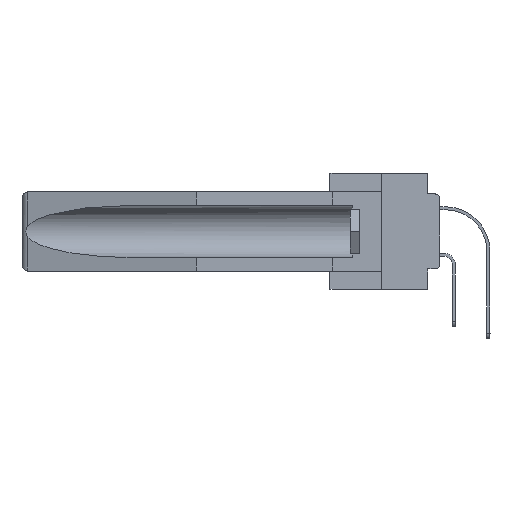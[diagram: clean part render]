
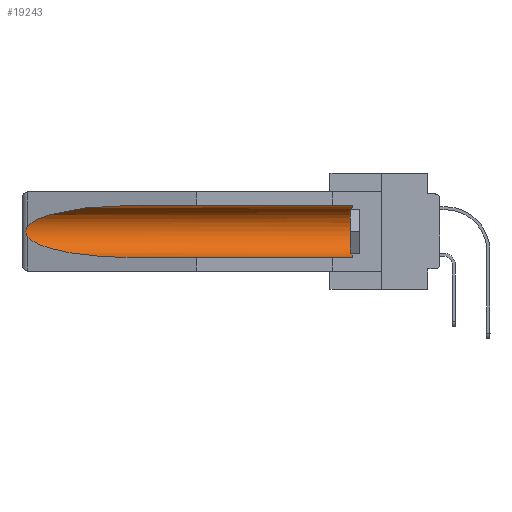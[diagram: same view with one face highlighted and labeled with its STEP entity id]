
A CAD part, left-side view. The second image highlights one B-rep face of the part: STEP entity #19243.
In plain terms, the highlighted cylindrical face has radius 2.857 mm (diameter 5.715 mm), a partial arc.
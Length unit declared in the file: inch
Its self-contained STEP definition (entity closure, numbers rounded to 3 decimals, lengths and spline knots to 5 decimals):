
#1200 = CARTESIAN_POINT ( 'NONE',  ( 0.155, 1.07973, -0.284 ) ) ;
#1222 = CARTESIAN_POINT ( 'NONE',  ( 0.2675, 1.53308, -0.16763 ) ) ;
#1404 = CARTESIAN_POINT ( 'NONE',  ( 0.26597, 1.5296, -0.19026 ) ) ;
#3200 = CARTESIAN_POINT ( 'NONE',  ( 0.26537, 1.52718, -0.19328 ) ) ;
#3252 = AXIS2_PLACEMENT_3D ( 'NONE', #8581, #19879, #29312 ) ;
#3478 =( BOUNDED_CURVE ( )  B_SPLINE_CURVE ( 3, ( #15281, #17588, #27032, #1200 ),
 .UNSPECIFIED., .F., .F. ) 
 B_SPLINE_CURVE_WITH_KNOTS ( ( 4, 4 ),
 ( 0.1948, 1.5708 ),
 .UNSPECIFIED. ) 
 CURVE ( )  GEOMETRIC_REPRESENTATION_ITEM ( )  RATIONAL_B_SPLINE_CURVE ( ( 1., 0.848, 0.848, 1. ) ) 
 REPRESENTATION_ITEM ( '' )  );
#4087 = CARTESIAN_POINT ( 'NONE',  ( 0.25451, 1.48313, -0.09465 ) ) ;
#4422 = AXIS2_PLACEMENT_3D ( 'NONE', #6371, #16258, #25703 ) ;
#4502 = EDGE_LOOP ( 'NONE', ( #12673, #25443, #23238, #27406, #7830, #9350 ) ) ;
#5231 = VECTOR ( 'NONE', #22722, 39.37008 ) ;
#5834 = LINE ( 'NONE', #6122, #15547 ) ;
#6122 = CARTESIAN_POINT ( 'NONE',  ( 0.155, -0.30754, -0.059 ) ) ;
#6148 = CARTESIAN_POINT ( 'NONE',  ( 0.155, -0.30754, -0.284 ) ) ;
#6371 = CARTESIAN_POINT ( 'NONE',  ( 0.155, -0.30754, -0.1715 ) ) ;
#6819 = CYLINDRICAL_SURFACE ( 'NONE', #4422, 0.1125 ) ;
#7031 = VERTEX_POINT ( 'NONE', #27412 ) ;
#7830 = ORIENTED_EDGE ( 'NONE', *, *, #12234, .T. ) ;
#7879 = CARTESIAN_POINT ( 'NONE',  ( 0.26537, 1.52718, -0.19328 ) ) ;
#8014 = VERTEX_POINT ( 'NONE', #3200 ) ;
#8350 = CARTESIAN_POINT ( 'NONE',  ( 0.2675, 1.53308, -0.17534 ) ) ;
#8578 = CARTESIAN_POINT ( 'NONE',  ( 0.155, 1.07973, -0.059 ) ) ;
#8581 = CARTESIAN_POINT ( 'NONE',  ( 0.155, 0.126, -0.1715 ) ) ;
#9350 = ORIENTED_EDGE ( 'NONE', *, *, #28765, .T. ) ;
#9729 = VERTEX_POINT ( 'NONE', #26986 ) ;
#10598 = EDGE_CURVE ( 'NONE', #8014, #28933, #3478, .T. ) ;
#11189 = EDGE_CURVE ( 'NONE', #9729, #14459, #22428, .T. ) ;
#12234 = EDGE_CURVE ( 'NONE', #7031, #19038, #16594, .T. ) ;
#12673 = ORIENTED_EDGE ( 'NONE', *, *, #11189, .T. ) ;
#12984 = CARTESIAN_POINT ( 'NONE',  ( 0.26654, 1.53092, -0.15636 ) ) ;
#13174 = CARTESIAN_POINT ( 'NONE',  ( 0.155, 0.126, -0.059 ) ) ;
#13753 = LINE ( 'NONE', #6148, #5231 ) ;
#13843 = CARTESIAN_POINT ( 'NONE',  ( 0.21114, 1.30732, -0.059 ) ) ;
#14004 = CARTESIAN_POINT ( 'NONE',  ( 0.155, 1.07973, -0.284 ) ) ;
#14459 = VERTEX_POINT ( 'NONE', #18401 ) ;
#15281 = CARTESIAN_POINT ( 'NONE',  ( 0.26537, 1.52718, -0.19328 ) ) ;
#15301 = CARTESIAN_POINT ( 'NONE',  ( 0.26537, 1.52718, -0.14972 ) ) ;
#15547 = VECTOR ( 'NONE', #27026, 39.37008 ) ;
#16258 = DIRECTION ( 'NONE',  ( 0., 1., 0. ) ) ;
#16287 = EDGE_CURVE ( 'NONE', #7031, #28933, #13753, .T. ) ;
#16594 = CIRCLE ( 'NONE', #3252, 0.1125 ) ;
#17588 = CARTESIAN_POINT ( 'NONE',  ( 0.25451, 1.48313, -0.24835 ) ) ;
#17781 = CARTESIAN_POINT ( 'NONE',  ( 0.2673, 1.53269, -0.17917 ) ) ;
#18401 = CARTESIAN_POINT ( 'NONE',  ( 0.26537, 1.52718, -0.14972 ) ) ;
#19038 = VERTEX_POINT ( 'NONE', #13174 ) ;
#19243 = ADVANCED_FACE ( 'NONE', ( #25094 ), #6819, .F. ) ;
#19569 = EDGE_CURVE ( 'NONE', #14459, #8014, #25384, .T. ) ;
#19879 = DIRECTION ( 'NONE',  ( 0., -1., 0. ) ) ;
#22401 = CARTESIAN_POINT ( 'NONE',  ( 0.26597, 1.52961, -0.15275 ) ) ;
#22428 =( BOUNDED_CURVE ( )  B_SPLINE_CURVE ( 3, ( #8578, #13843, #4087, #23122 ),
 .UNSPECIFIED., .F., .F. ) 
 B_SPLINE_CURVE_WITH_KNOTS ( ( 4, 4 ),
 ( 4.71239, 6.08839 ),
 .UNSPECIFIED. ) 
 CURVE ( )  GEOMETRIC_REPRESENTATION_ITEM ( )  RATIONAL_B_SPLINE_CURVE ( ( 1., 0.848, 0.848, 1. ) ) 
 REPRESENTATION_ITEM ( '' )  );
#22556 = CARTESIAN_POINT ( 'NONE',  ( 0.26655, 1.53094, -0.18657 ) ) ;
#22722 = DIRECTION ( 'NONE',  ( 0., 1., 0. ) ) ;
#23122 = CARTESIAN_POINT ( 'NONE',  ( 0.26537, 1.52718, -0.14972 ) ) ;
#23238 = ORIENTED_EDGE ( 'NONE', *, *, #10598, .T. ) ;
#24739 = CARTESIAN_POINT ( 'NONE',  ( 0.2673, 1.5327, -0.16383 ) ) ;
#25094 = FACE_OUTER_BOUND ( 'NONE', #4502, .T. ) ;
#25384 = B_SPLINE_CURVE_WITH_KNOTS ( 'NONE', 3,
 ( #15301, #22401, #12984, #24739, #1222, #8350, #17781, #22556, #1404, #7879 ),
 .UNSPECIFIED., .F., .F.,
 ( 4, 2, 2, 2, 4 ),
 ( 0., 0.00029, 0.00058, 0.00087, 0.00117 ),
 .UNSPECIFIED. ) ;
#25443 = ORIENTED_EDGE ( 'NONE', *, *, #19569, .T. ) ;
#25703 = DIRECTION ( 'NONE',  ( 0., 0., 1. ) ) ;
#26986 = CARTESIAN_POINT ( 'NONE',  ( 0.155, 1.07973, -0.059 ) ) ;
#27026 = DIRECTION ( 'NONE',  ( 0., 1., 0. ) ) ;
#27032 = CARTESIAN_POINT ( 'NONE',  ( 0.21114, 1.30732, -0.284 ) ) ;
#27406 = ORIENTED_EDGE ( 'NONE', *, *, #16287, .F. ) ;
#27412 = CARTESIAN_POINT ( 'NONE',  ( 0.155, 0.126, -0.284 ) ) ;
#28765 = EDGE_CURVE ( 'NONE', #19038, #9729, #5834, .T. ) ;
#28933 = VERTEX_POINT ( 'NONE', #14004 ) ;
#29312 = DIRECTION ( 'NONE',  ( 0., 0., 1. ) ) ;
